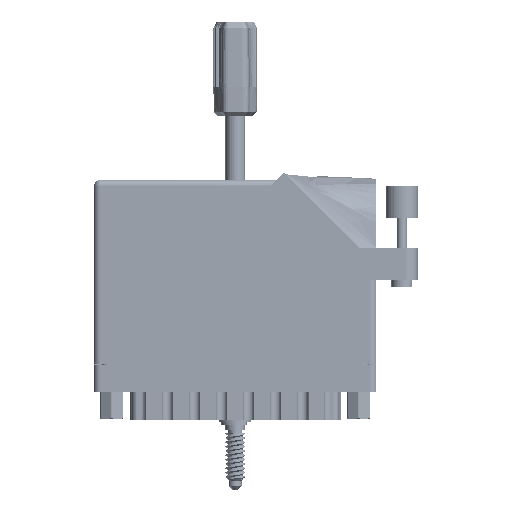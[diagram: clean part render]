
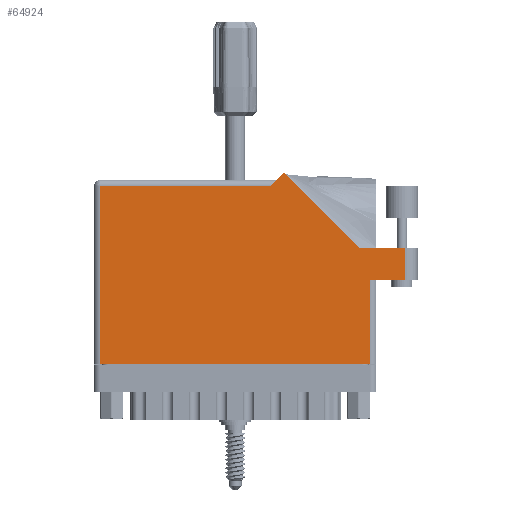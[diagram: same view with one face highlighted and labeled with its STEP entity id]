
A CAD part, front view. The second image highlights one B-rep face of the part: STEP entity #64924.
In plain terms, the highlighted face is planar.
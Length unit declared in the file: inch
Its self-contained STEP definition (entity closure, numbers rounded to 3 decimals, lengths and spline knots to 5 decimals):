
#152 = DIRECTION ( 'NONE',  ( -1., 0., 0. ) ) ;
#314 = LINE ( 'NONE', #67476, #27684 ) ;
#480 = VECTOR ( 'NONE', #80854, 39.37008 ) ;
#1008 = VECTOR ( 'NONE', #93994, 39.37008 ) ;
#1475 = EDGE_CURVE ( 'NONE', #6277, #3925, #41370, .T. ) ;
#3774 = DIRECTION ( 'NONE',  ( 0., 1., 0. ) ) ;
#3925 = VERTEX_POINT ( 'NONE', #60992 ) ;
#6209 = CARTESIAN_POINT ( 'NONE',  ( 2.55242, 1.122, 0. ) ) ;
#6277 = VERTEX_POINT ( 'NONE', #57834 ) ;
#7978 = EDGE_CURVE ( 'NONE', #30612, #40539, #81766, .T. ) ;
#10981 = DIRECTION ( 'NONE',  ( 0., 1., 0. ) ) ;
#11204 = VERTEX_POINT ( 'NONE', #35964 ) ;
#14305 = CARTESIAN_POINT ( 'NONE',  ( 0.062, 0., 0. ) ) ;
#17159 = VECTOR ( 'NONE', #91561, 39.37008 ) ;
#17190 = PLANE ( 'NONE',  #51731 ) ;
#17292 = ORIENTED_EDGE ( 'NONE', *, *, #41215, .T. ) ;
#18291 = LINE ( 'NONE', #92521, #1008 ) ;
#19723 = CARTESIAN_POINT ( 'NONE',  ( 3.118, 1.122, 0. ) ) ;
#19951 = ORIENTED_EDGE ( 'NONE', *, *, #51320, .T. ) ;
#23216 = FACE_OUTER_BOUND ( 'NONE', #55158, .T. ) ;
#25097 = VECTOR ( 'NONE', #3774, 39.37008 ) ;
#26341 = CARTESIAN_POINT ( 'NONE',  ( 2.993, 1.122, 0. ) ) ;
#27684 = VECTOR ( 'NONE', #67966, 39.37008 ) ;
#29219 = CARTESIAN_POINT ( 'NONE',  ( 2.718, 0.815, 0. ) ) ;
#29820 = CARTESIAN_POINT ( 'NONE',  ( 0.062, 1.713, 0. ) ) ;
#30163 = EDGE_CURVE ( 'NONE', #67282, #94419, #314, .T. ) ;
#30612 = VERTEX_POINT ( 'NONE', #6209 ) ;
#31802 = EDGE_CURVE ( 'NONE', #11204, #67282, #68752, .T. ) ;
#34068 = CARTESIAN_POINT ( 'NONE',  ( 2.656, 0., 0. ) ) ;
#35964 = CARTESIAN_POINT ( 'NONE',  ( 1.696, 1.713, 0. ) ) ;
#37218 = ORIENTED_EDGE ( 'NONE', *, *, #7978, .T. ) ;
#39413 = CARTESIAN_POINT ( 'NONE',  ( 0., 0., 0. ) ) ;
#40539 = VERTEX_POINT ( 'NONE', #83343 ) ;
#41059 = LINE ( 'NONE', #63142, #89383 ) ;
#41215 = EDGE_CURVE ( 'NONE', #40539, #11204, #18291, .T. ) ;
#41370 = LINE ( 'NONE', #26341, #25097 ) ;
#43473 = ORIENTED_EDGE ( 'NONE', *, *, #31802, .T. ) ;
#43564 = EDGE_CURVE ( 'NONE', #58536, #91956, #41059, .T. ) ;
#45948 = LINE ( 'NONE', #39413, #17159 ) ;
#46271 = CARTESIAN_POINT ( 'NONE',  ( 0., 1.775, 0. ) ) ;
#47745 = DIRECTION ( 'NONE',  ( 0., 0., -1. ) ) ;
#51320 = EDGE_CURVE ( 'NONE', #3925, #30612, #88863, .T. ) ;
#51731 = AXIS2_PLACEMENT_3D ( 'NONE', #46271, #47745, #152 ) ;
#51748 = DIRECTION ( 'NONE',  ( 1., 0., 0. ) ) ;
#55158 = EDGE_LOOP ( 'NONE', ( #72506, #87571, #19951, #37218, #17292, #43473, #81892, #85587, #62746 ) ) ;
#57834 = CARTESIAN_POINT ( 'NONE',  ( 2.993, 0.815, 0. ) ) ;
#58536 = VERTEX_POINT ( 'NONE', #34068 ) ;
#60992 = CARTESIAN_POINT ( 'NONE',  ( 2.993, 1.122, 0. ) ) ;
#61227 = DIRECTION ( 'NONE',  ( -1., 0., 0. ) ) ;
#61294 = LINE ( 'NONE', #29219, #87214 ) ;
#62746 = ORIENTED_EDGE ( 'NONE', *, *, #43564, .T. ) ;
#63142 = CARTESIAN_POINT ( 'NONE',  ( 2.656, 0.815, 0. ) ) ;
#64924 = ADVANCED_FACE ( 'NONE', ( #23216 ), #17190, .F. ) ;
#66252 = CARTESIAN_POINT ( 'NONE',  ( 2.55242, 1.122, 0. ) ) ;
#66550 = CARTESIAN_POINT ( 'NONE',  ( 2.656, 0.815, 0. ) ) ;
#67282 = VERTEX_POINT ( 'NONE', #29820 ) ;
#67476 = CARTESIAN_POINT ( 'NONE',  ( 0.062, 0., 0. ) ) ;
#67966 = DIRECTION ( 'NONE',  ( 0., -1., 0. ) ) ;
#68752 = LINE ( 'NONE', #74765, #91169 ) ;
#70786 = EDGE_CURVE ( 'NONE', #94419, #58536, #45948, .T. ) ;
#72506 = ORIENTED_EDGE ( 'NONE', *, *, #94895, .T. ) ;
#74765 = CARTESIAN_POINT ( 'NONE',  ( 0., 1.713, 0. ) ) ;
#80854 = DIRECTION ( 'NONE',  ( -1., 0., 0. ) ) ;
#81766 = LINE ( 'NONE', #66252, #97242 ) ;
#81892 = ORIENTED_EDGE ( 'NONE', *, *, #30163, .T. ) ;
#83343 = CARTESIAN_POINT ( 'NONE',  ( 1.82871, 1.84571, 0. ) ) ;
#85587 = ORIENTED_EDGE ( 'NONE', *, *, #70786, .T. ) ;
#87214 = VECTOR ( 'NONE', #51748, 39.37008 ) ;
#87571 = ORIENTED_EDGE ( 'NONE', *, *, #1475, .T. ) ;
#88863 = LINE ( 'NONE', #19723, #480 ) ;
#89383 = VECTOR ( 'NONE', #10981, 39.37008 ) ;
#91169 = VECTOR ( 'NONE', #61227, 39.37008 ) ;
#91561 = DIRECTION ( 'NONE',  ( 1., 0., 0. ) ) ;
#91956 = VERTEX_POINT ( 'NONE', #66550 ) ;
#92521 = CARTESIAN_POINT ( 'NONE',  ( 1.758, 1.775, 0. ) ) ;
#93994 = DIRECTION ( 'NONE',  ( -0.707, -0.707, 0. ) ) ;
#94419 = VERTEX_POINT ( 'NONE', #14305 ) ;
#94895 = EDGE_CURVE ( 'NONE', #91956, #6277, #61294, .T. ) ;
#95837 = DIRECTION ( 'NONE',  ( -0.707, 0.707, 0. ) ) ;
#97242 = VECTOR ( 'NONE', #95837, 39.37008 ) ;
